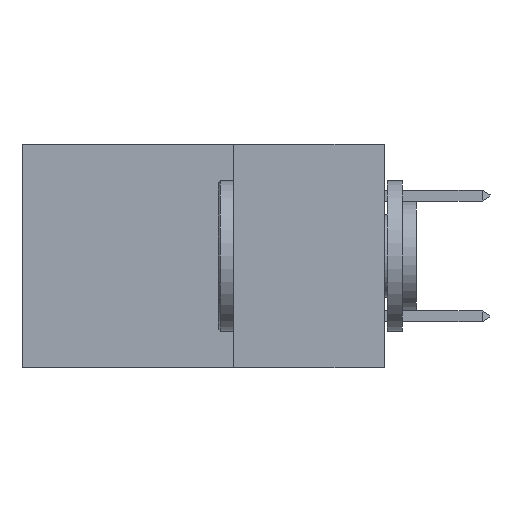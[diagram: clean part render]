
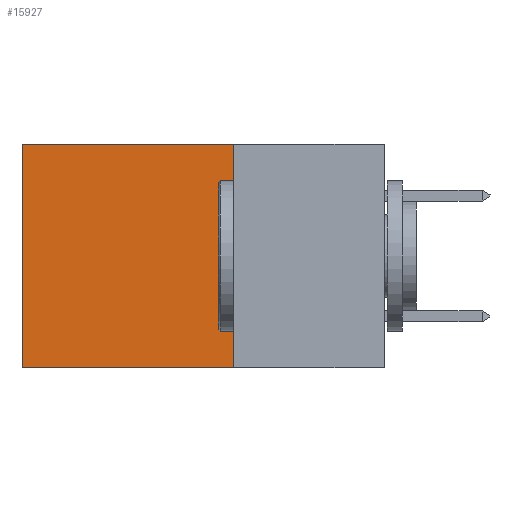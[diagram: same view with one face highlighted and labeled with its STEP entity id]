
A CAD part, left-side view. The second image highlights one B-rep face of the part: STEP entity #15927.
In plain terms, the highlighted planar face has unit normal (-1, 0, 0).
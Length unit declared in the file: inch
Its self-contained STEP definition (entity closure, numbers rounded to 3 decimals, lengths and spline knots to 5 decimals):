
#1086 = CARTESIAN_POINT ( 'NONE',  ( 0.2875, 0.25, 0. ) ) ;
#1294 = EDGE_CURVE ( 'NONE', #14623, #21860, #20399, .T. ) ;
#2583 = ORIENTED_EDGE ( 'NONE', *, *, #24420, .T. ) ;
#3832 = DIRECTION ( 'NONE',  ( 0., 0., -1. ) ) ;
#5651 = DIRECTION ( 'NONE',  ( 1., 0., 0. ) ) ;
#7058 = CARTESIAN_POINT ( 'NONE',  ( 0.2875, 0.25, 0. ) ) ;
#7782 = VECTOR ( 'NONE', #21020, 39.37008 ) ;
#9565 = VERTEX_POINT ( 'NONE', #17084 ) ;
#10265 = EDGE_LOOP ( 'NONE', ( #2583, #14322, #11322, #28801 ) ) ;
#11105 = DIRECTION ( 'NONE',  ( 0., 0., -1. ) ) ;
#11322 = ORIENTED_EDGE ( 'NONE', *, *, #24551, .F. ) ;
#12233 = PLANE ( 'NONE',  #24634 ) ;
#12727 = VECTOR ( 'NONE', #3832, 39.37008 ) ;
#13424 = LINE ( 'NONE', #26376, #12727 ) ;
#14322 = ORIENTED_EDGE ( 'NONE', *, *, #1294, .F. ) ;
#14623 = VERTEX_POINT ( 'NONE', #14829 ) ;
#14829 = CARTESIAN_POINT ( 'NONE',  ( 0.2875, 0.25, -0.37 ) ) ;
#15160 = LINE ( 'NONE', #24582, #15870 ) ;
#15608 = CARTESIAN_POINT ( 'NONE',  ( 0.2875, 0.25, 0. ) ) ;
#15870 = VECTOR ( 'NONE', #11105, 39.37008 ) ;
#15927 = ADVANCED_FACE ( 'NONE', ( #19524 ), #12233, .F. ) ;
#16508 = CARTESIAN_POINT ( 'NONE',  ( 0.2875, 0.25, -0.37 ) ) ;
#16869 = CARTESIAN_POINT ( 'NONE',  ( 0.2875, 0.6, -0.37 ) ) ;
#17084 = CARTESIAN_POINT ( 'NONE',  ( 0.2875, 0.6, 0. ) ) ;
#19524 = FACE_OUTER_BOUND ( 'NONE', #10265, .T. ) ;
#20399 = LINE ( 'NONE', #16508, #7782 ) ;
#21020 = DIRECTION ( 'NONE',  ( 0., 1., 0. ) ) ;
#21356 = DIRECTION ( 'NONE',  ( 0., 0., -1. ) ) ;
#21860 = VERTEX_POINT ( 'NONE', #16869 ) ;
#23515 = LINE ( 'NONE', #7058, #28826 ) ;
#24420 = EDGE_CURVE ( 'NONE', #9565, #21860, #13424, .T. ) ;
#24551 = EDGE_CURVE ( 'NONE', #24581, #14623, #15160, .T. ) ;
#24581 = VERTEX_POINT ( 'NONE', #15608 ) ;
#24582 = CARTESIAN_POINT ( 'NONE',  ( 0.2875, 0.25, 0. ) ) ;
#24634 = AXIS2_PLACEMENT_3D ( 'NONE', #1086, #5651, #21356 ) ;
#25041 = DIRECTION ( 'NONE',  ( 0., 1., 0. ) ) ;
#26376 = CARTESIAN_POINT ( 'NONE',  ( 0.2875, 0.6, 0. ) ) ;
#28801 = ORIENTED_EDGE ( 'NONE', *, *, #29179, .T. ) ;
#28826 = VECTOR ( 'NONE', #25041, 39.37008 ) ;
#29179 = EDGE_CURVE ( 'NONE', #24581, #9565, #23515, .T. ) ;
